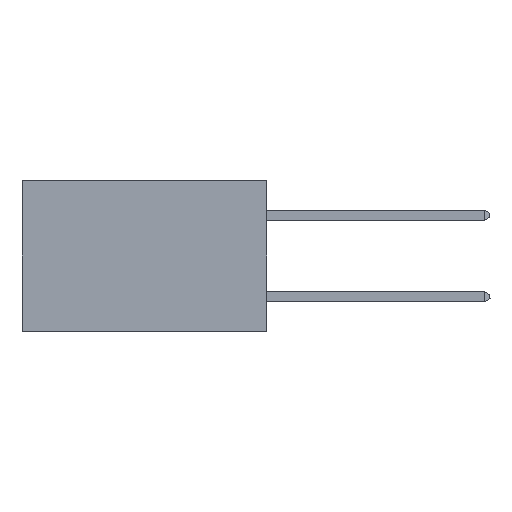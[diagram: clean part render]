
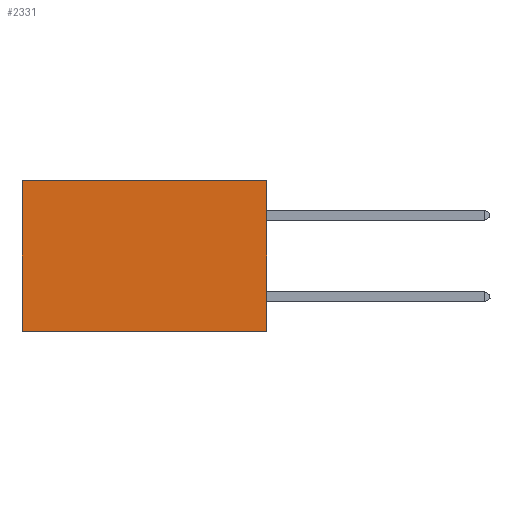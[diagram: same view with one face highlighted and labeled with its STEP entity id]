
A CAD part, left-side view. The second image highlights one B-rep face of the part: STEP entity #2331.
In plain terms, the highlighted planar face has unit normal (-1, 0, 0).
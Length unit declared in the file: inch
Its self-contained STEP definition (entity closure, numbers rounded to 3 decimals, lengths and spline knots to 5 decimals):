
#1787 = DIRECTION ( 'NONE',  ( 0., 0., -1. ) ) ;
#2331 = ADVANCED_FACE ( 'NONE', ( #7450 ), #7540, .F. ) ;
#2839 = CARTESIAN_POINT ( 'NONE',  ( 0.2875, 0., -0.37 ) ) ;
#4289 = VERTEX_POINT ( 'NONE', #6420 ) ;
#4746 = CARTESIAN_POINT ( 'NONE',  ( 0.2875, 0., 0. ) ) ;
#5954 = DIRECTION ( 'NONE',  ( 0., 0., -1. ) ) ;
#6010 = CARTESIAN_POINT ( 'NONE',  ( 0.2875, 0., -0.37 ) ) ;
#6257 = CARTESIAN_POINT ( 'NONE',  ( 0.2875, 0.6, -0.37 ) ) ;
#6420 = CARTESIAN_POINT ( 'NONE',  ( 0.2875, 0., 0. ) ) ;
#6553 = LINE ( 'NONE', #14718, #29099 ) ;
#6648 = AXIS2_PLACEMENT_3D ( 'NONE', #4746, #15082, #7771 ) ;
#7450 = FACE_OUTER_BOUND ( 'NONE', #22722, .T. ) ;
#7540 = PLANE ( 'NONE',  #6648 ) ;
#7771 = DIRECTION ( 'NONE',  ( 0., 0., -1. ) ) ;
#10694 = LINE ( 'NONE', #20610, #24833 ) ;
#10974 = EDGE_CURVE ( 'NONE', #4289, #30396, #10694, .T. ) ;
#11781 = LINE ( 'NONE', #23844, #14568 ) ;
#13211 = VERTEX_POINT ( 'NONE', #6257 ) ;
#13238 = DIRECTION ( 'NONE',  ( 0., 1., 0. ) ) ;
#14459 = LINE ( 'NONE', #6010, #15627 ) ;
#14568 = VECTOR ( 'NONE', #13238, 39.37008 ) ;
#14718 = CARTESIAN_POINT ( 'NONE',  ( 0.2875, 0.6, 0. ) ) ;
#15082 = DIRECTION ( 'NONE',  ( 1., 0., 0. ) ) ;
#15627 = VECTOR ( 'NONE', #27142, 39.37008 ) ;
#17478 = CARTESIAN_POINT ( 'NONE',  ( 0.2875, 0.6, 0. ) ) ;
#17770 = ORIENTED_EDGE ( 'NONE', *, *, #28166, .T. ) ;
#18424 = EDGE_CURVE ( 'NONE', #30396, #13211, #14459, .T. ) ;
#20300 = ORIENTED_EDGE ( 'NONE', *, *, #28276, .T. ) ;
#20610 = CARTESIAN_POINT ( 'NONE',  ( 0.2875, 0., 0. ) ) ;
#20850 = VERTEX_POINT ( 'NONE', #17478 ) ;
#22722 = EDGE_LOOP ( 'NONE', ( #20300, #25694, #25374, #17770 ) ) ;
#23844 = CARTESIAN_POINT ( 'NONE',  ( 0.2875, 0., 0. ) ) ;
#24833 = VECTOR ( 'NONE', #5954, 39.37008 ) ;
#25374 = ORIENTED_EDGE ( 'NONE', *, *, #10974, .F. ) ;
#25694 = ORIENTED_EDGE ( 'NONE', *, *, #18424, .F. ) ;
#27142 = DIRECTION ( 'NONE',  ( 0., 1., 0. ) ) ;
#28166 = EDGE_CURVE ( 'NONE', #4289, #20850, #11781, .T. ) ;
#28276 = EDGE_CURVE ( 'NONE', #20850, #13211, #6553, .T. ) ;
#29099 = VECTOR ( 'NONE', #1787, 39.37008 ) ;
#30396 = VERTEX_POINT ( 'NONE', #2839 ) ;
